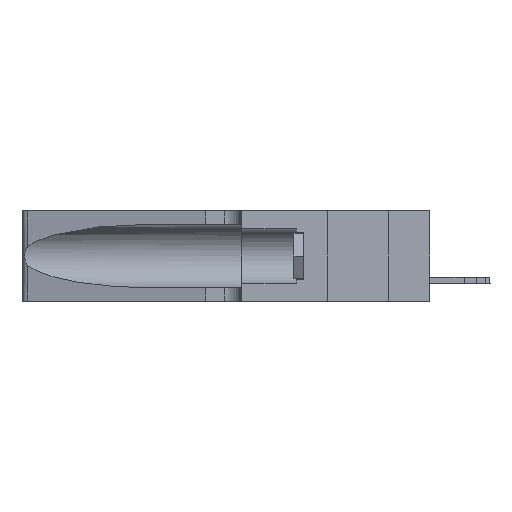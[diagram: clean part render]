
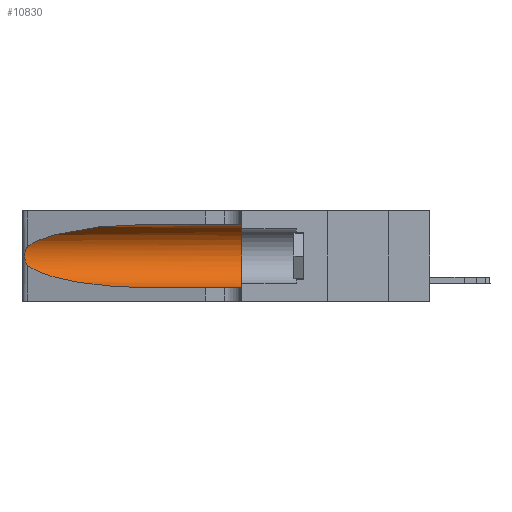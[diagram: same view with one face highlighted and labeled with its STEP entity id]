
A CAD part, left-side view. The second image highlights one B-rep face of the part: STEP entity #10830.
In plain terms, the highlighted cylindrical face has radius 3.308 mm (diameter 6.617 mm), a partial arc.
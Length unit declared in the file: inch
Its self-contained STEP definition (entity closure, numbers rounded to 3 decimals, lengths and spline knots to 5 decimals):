
#380 = EDGE_LOOP ( 'NONE', ( #11391, #7757, #9916, #5661, #2941, #1152 ) ) ;
#434 = CARTESIAN_POINT ( 'NONE',  ( 0.1305, 0.72297, 0.31525 ) ) ;
#516 = CARTESIAN_POINT ( 'NONE',  ( 0.18966, 0.96281, 0.31525 ) ) ;
#961 = CARTESIAN_POINT ( 'NONE',  ( 0.1305, 0.35, 0.05475 ) ) ;
#1152 = ORIENTED_EDGE ( 'NONE', *, *, #2108, .F. ) ;
#1708 = LINE ( 'NONE', #16307, #7244 ) ;
#1755 = LINE ( 'NONE', #17760, #15966 ) ;
#2108 = EDGE_CURVE ( 'NONE', #3947, #13494, #1755, .T. ) ;
#2342 = DIRECTION ( 'NONE',  ( 0., 0., -1. ) ) ;
#2354 = CARTESIAN_POINT ( 'NONE',  ( 0.1305, 0.72297, 0.05475 ) ) ;
#2941 = ORIENTED_EDGE ( 'NONE', *, *, #4369, .F. ) ;
#3034 = FACE_OUTER_BOUND ( 'NONE', #380, .T. ) ;
#3395 =( BOUNDED_CURVE ( )  B_SPLINE_CURVE ( 3, ( #434, #516, #9973, #8238 ),
 .UNSPECIFIED., .F., .F. ) 
 B_SPLINE_CURVE_WITH_KNOTS ( ( 4, 4 ),
 ( 1.5708, 2.84003 ),
 .UNSPECIFIED. ) 
 CURVE ( )  GEOMETRIC_REPRESENTATION_ITEM ( )  RATIONAL_B_SPLINE_CURVE ( ( 1., 0.87, 0.87, 1. ) ) 
 REPRESENTATION_ITEM ( '' )  );
#3496 = CARTESIAN_POINT ( 'NONE',  ( 0.25789, 1.23486, 0.15765 ) ) ;
#3947 = VERTEX_POINT ( 'NONE', #16639 ) ;
#4369 = EDGE_CURVE ( 'NONE', #13494, #14613, #23042, .T. ) ;
#5317 = AXIS2_PLACEMENT_3D ( 'NONE', #9629, #7972, #5853 ) ;
#5661 = ORIENTED_EDGE ( 'NONE', *, *, #18300, .T. ) ;
#5853 = DIRECTION ( 'NONE',  ( 0., 0., 1. ) ) ;
#6804 = VERTEX_POINT ( 'NONE', #14986 ) ;
#7102 = CARTESIAN_POINT ( 'NONE',  ( 0.26018, 1.23835, 0.19895 ) ) ;
#7221 = CARTESIAN_POINT ( 'NONE',  ( 0.18966, 0.96281, 0.05475 ) ) ;
#7244 = VECTOR ( 'NONE', #10608, 39.37008 ) ;
#7757 = ORIENTED_EDGE ( 'NONE', *, *, #11865, .T. ) ;
#7972 = DIRECTION ( 'NONE',  ( 0., 1., 0. ) ) ;
#8178 = CARTESIAN_POINT ( 'NONE',  ( 0.1305, 0.35, 0.31525 ) ) ;
#8238 = CARTESIAN_POINT ( 'NONE',  ( 0.25487, 1.22718, 0.22369 ) ) ;
#8583 = CARTESIAN_POINT ( 'NONE',  ( 0.25487, 1.22718, 0.22369 ) ) ;
#8901 = DIRECTION ( 'NONE',  ( 0., -1., 0. ) ) ;
#9148 = CARTESIAN_POINT ( 'NONE',  ( 0.26075, 1.23896, 0.19203 ) ) ;
#9629 = CARTESIAN_POINT ( 'NONE',  ( 0.1305, 0.35, 0.185 ) ) ;
#9916 = ORIENTED_EDGE ( 'NONE', *, *, #11105, .T. ) ;
#9973 = CARTESIAN_POINT ( 'NONE',  ( 0.2373, 1.15595, 0.28018 ) ) ;
#10608 = DIRECTION ( 'NONE',  ( 0., -1., 0. ) ) ;
#10830 = ADVANCED_FACE ( 'NONE', ( #3034 ), #15519, .F. ) ;
#10911 = CARTESIAN_POINT ( 'NONE',  ( 0.2373, 1.15595, 0.08982 ) ) ;
#11105 = EDGE_CURVE ( 'NONE', #6804, #13827, #18263, .T. ) ;
#11391 = ORIENTED_EDGE ( 'NONE', *, *, #22177, .T. ) ;
#11865 = EDGE_CURVE ( 'NONE', #21864, #6804, #20759, .T. ) ;
#12879 = CARTESIAN_POINT ( 'NONE',  ( 0.25555, 1.22993, 0.14849 ) ) ;
#13494 = VERTEX_POINT ( 'NONE', #8178 ) ;
#13827 = VERTEX_POINT ( 'NONE', #2354 ) ;
#14388 = CARTESIAN_POINT ( 'NONE',  ( 0.25639, 1.23184, 0.21858 ) ) ;
#14464 = CARTESIAN_POINT ( 'NONE',  ( 0.25787, 1.23484, 0.2124 ) ) ;
#14613 = VERTEX_POINT ( 'NONE', #961 ) ;
#14986 = CARTESIAN_POINT ( 'NONE',  ( 0.25487, 1.22718, 0.14631 ) ) ;
#15519 = CYLINDRICAL_SURFACE ( 'NONE', #17516, 0.13025 ) ;
#15966 = VECTOR ( 'NONE', #8901, 39.37008 ) ;
#16307 = CARTESIAN_POINT ( 'NONE',  ( 0.1305, 1.61858, 0.05475 ) ) ;
#16393 = CARTESIAN_POINT ( 'NONE',  ( 0.26017, 1.23833, 0.17102 ) ) ;
#16639 = CARTESIAN_POINT ( 'NONE',  ( 0.1305, 0.72297, 0.31525 ) ) ;
#17516 = AXIS2_PLACEMENT_3D ( 'NONE', #20629, #18876, #2342 ) ;
#17760 = CARTESIAN_POINT ( 'NONE',  ( 0.1305, 1.61858, 0.31525 ) ) ;
#18167 = CARTESIAN_POINT ( 'NONE',  ( 0.25555, 1.22994, 0.2215 ) ) ;
#18239 = CARTESIAN_POINT ( 'NONE',  ( 0.25854, 1.2359, 0.20912 ) ) ;
#18263 =( BOUNDED_CURVE ( )  B_SPLINE_CURVE ( 3, ( #20038, #10911, #7221, #23674 ),
 .UNSPECIFIED., .F., .T. ) 
 B_SPLINE_CURVE_WITH_KNOTS ( ( 4, 4 ),
 ( 3.44316, 4.71239 ),
 .UNSPECIFIED. ) 
 CURVE ( )  GEOMETRIC_REPRESENTATION_ITEM ( )  RATIONAL_B_SPLINE_CURVE ( ( 1., 0.87, 0.87, 1. ) ) 
 REPRESENTATION_ITEM ( '' )  );
#18300 = EDGE_CURVE ( 'NONE', #13827, #14613, #1708, .T. ) ;
#18876 = DIRECTION ( 'NONE',  ( 0., -1., 0. ) ) ;
#19998 = CARTESIAN_POINT ( 'NONE',  ( 0.26075, 1.23896, 0.178 ) ) ;
#20038 = CARTESIAN_POINT ( 'NONE',  ( 0.25487, 1.22718, 0.14631 ) ) ;
#20164 = CARTESIAN_POINT ( 'NONE',  ( 0.25487, 1.22718, 0.22369 ) ) ;
#20629 = CARTESIAN_POINT ( 'NONE',  ( 0.1305, 1.61858, 0.185 ) ) ;
#20759 = B_SPLINE_CURVE_WITH_KNOTS ( 'NONE', 3,
 ( #20164, #18167, #14388, #14464, #18239, #7102, #9148, #19998, #16393, #22017, #3496, #21865, #12879, #23712 ),
 .UNSPECIFIED., .F., .F.,
 ( 4, 2, 2, 2, 2, 2, 4 ),
 ( 0., 0.00027, 0.00053, 0.00107, 0.0016, 0.00187, 0.00214 ),
 .UNSPECIFIED. ) ;
#21864 = VERTEX_POINT ( 'NONE', #8583 ) ;
#21865 = CARTESIAN_POINT ( 'NONE',  ( 0.25639, 1.23186, 0.15144 ) ) ;
#22017 = CARTESIAN_POINT ( 'NONE',  ( 0.25856, 1.23593, 0.16098 ) ) ;
#22177 = EDGE_CURVE ( 'NONE', #3947, #21864, #3395, .T. ) ;
#23042 = CIRCLE ( 'NONE', #5317, 0.13025 ) ;
#23674 = CARTESIAN_POINT ( 'NONE',  ( 0.1305, 0.72297, 0.05475 ) ) ;
#23712 = CARTESIAN_POINT ( 'NONE',  ( 0.25487, 1.22718, 0.14631 ) ) ;
